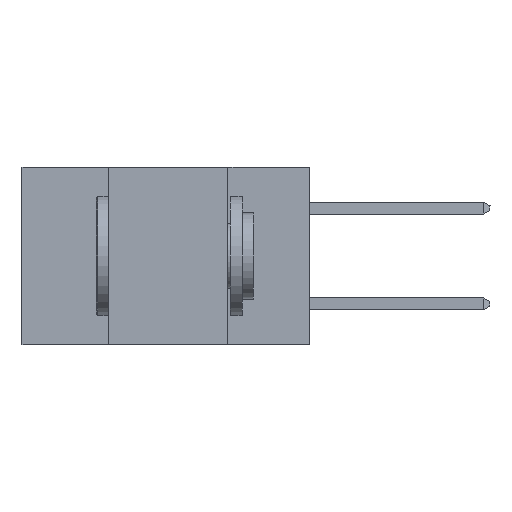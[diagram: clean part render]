
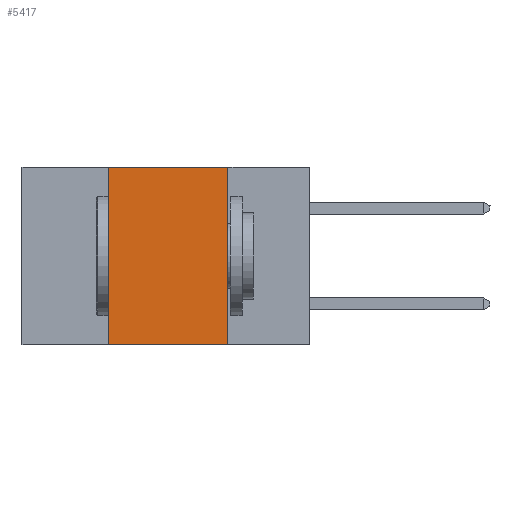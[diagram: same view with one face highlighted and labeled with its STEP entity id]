
A CAD part, left-side view. The second image highlights one B-rep face of the part: STEP entity #5417.
In plain terms, the highlighted planar face has unit normal (-1, 0, 0).
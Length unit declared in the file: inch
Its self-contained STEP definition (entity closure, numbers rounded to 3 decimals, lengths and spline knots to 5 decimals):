
#1434 = CARTESIAN_POINT ( 'NONE',  ( 0., 0.6, 0. ) ) ;
#2392 = DIRECTION ( 'NONE',  ( 1., 0., 0. ) ) ;
#3129 = VERTEX_POINT ( 'NONE', #26620 ) ;
#4106 = EDGE_CURVE ( 'NONE', #6636, #3129, #24174, .T. ) ;
#4856 = DIRECTION ( 'NONE',  ( 0., -1., 0. ) ) ;
#5417 = ADVANCED_FACE ( 'NONE', ( #16249 ), #30165, .F. ) ;
#6417 = CARTESIAN_POINT ( 'NONE',  ( 0., 0.42, -0.37 ) ) ;
#6636 = VERTEX_POINT ( 'NONE', #6417 ) ;
#7264 = EDGE_LOOP ( 'NONE', ( #17192, #9835, #19393, #18155 ) ) ;
#7632 = CARTESIAN_POINT ( 'NONE',  ( 0., 0.6, 0. ) ) ;
#9589 = LINE ( 'NONE', #28433, #28532 ) ;
#9835 = ORIENTED_EDGE ( 'NONE', *, *, #12294, .F. ) ;
#12294 = EDGE_CURVE ( 'NONE', #35312, #32615, #36012, .T. ) ;
#12336 = DIRECTION ( 'NONE',  ( 0., -1., 0. ) ) ;
#15641 = CARTESIAN_POINT ( 'NONE',  ( 0., 0.6, -0.37 ) ) ;
#16123 = DIRECTION ( 'NONE',  ( 0., 0., -1. ) ) ;
#16249 = FACE_OUTER_BOUND ( 'NONE', #7264, .T. ) ;
#17192 = ORIENTED_EDGE ( 'NONE', *, *, #31690, .F. ) ;
#18155 = ORIENTED_EDGE ( 'NONE', *, *, #4106, .T. ) ;
#19393 = ORIENTED_EDGE ( 'NONE', *, *, #23043, .F. ) ;
#19954 = DIRECTION ( 'NONE',  ( 0., 0., -1. ) ) ;
#23043 = EDGE_CURVE ( 'NONE', #6636, #35312, #9589, .T. ) ;
#24174 = LINE ( 'NONE', #15641, #36069 ) ;
#25704 = CARTESIAN_POINT ( 'NONE',  ( 0., 0.42, 0. ) ) ;
#25867 = CARTESIAN_POINT ( 'NONE',  ( 0., 0.17, 0. ) ) ;
#26620 = CARTESIAN_POINT ( 'NONE',  ( 0., 0.17, -0.37 ) ) ;
#28244 = LINE ( 'NONE', #25867, #32186 ) ;
#28433 = CARTESIAN_POINT ( 'NONE',  ( 0., 0.42, 0. ) ) ;
#28532 = VECTOR ( 'NONE', #28785, 39.37008 ) ;
#28785 = DIRECTION ( 'NONE',  ( 0., 0., 1. ) ) ;
#29379 = CARTESIAN_POINT ( 'NONE',  ( 0., 0.17, 0. ) ) ;
#30165 = PLANE ( 'NONE',  #34635 ) ;
#31690 = EDGE_CURVE ( 'NONE', #32615, #3129, #28244, .T. ) ;
#32186 = VECTOR ( 'NONE', #19954, 39.37008 ) ;
#32615 = VERTEX_POINT ( 'NONE', #29379 ) ;
#34635 = AXIS2_PLACEMENT_3D ( 'NONE', #7632, #2392, #16123 ) ;
#35092 = VECTOR ( 'NONE', #4856, 39.37008 ) ;
#35312 = VERTEX_POINT ( 'NONE', #25704 ) ;
#36012 = LINE ( 'NONE', #1434, #35092 ) ;
#36069 = VECTOR ( 'NONE', #12336, 39.37008 ) ;
